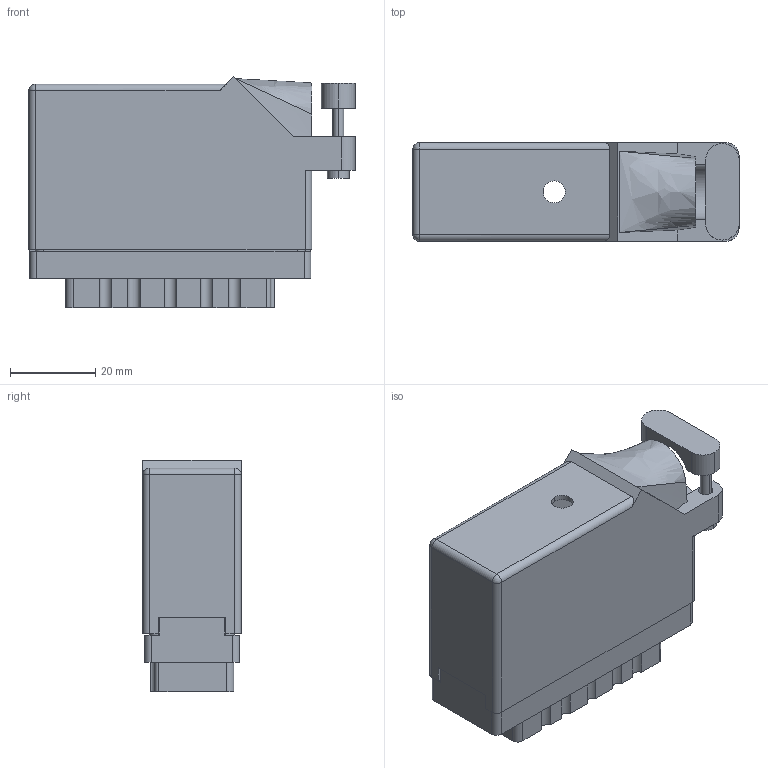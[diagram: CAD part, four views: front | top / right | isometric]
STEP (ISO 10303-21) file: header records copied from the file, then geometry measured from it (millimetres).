
FILE_DESCRIPTION (( 'STEP AP203' ), '1' );
FILE_NAME ('516-056-000-220.STEP', '2020-03-05T19:26:28', ( '' ), ( '' ), 'SwSTEP 2.0', 'SolidWorks 2016', '' );
FILE_SCHEMA (( 'CONFIG_CONTROL_DESIGN' ));
Length unit declared in the file: inch
Products named in the file (3): 516-056-000-220; 516-230-001_Plastic - 056 Side Entry; 516 Part Receptacle_056
Assembly tree (2 placements, depth 2):
  516-056-000-220
    516 Part Receptacle_056
    516-230-001_Plastic - 056 Side Entry
Bounding box: 76.5 x 23.11 x 54.15 mm (x, y, z)
Volume: 26495.7 mm3; surface area: 36846.7 mm2
Topology: 2 solids, 2 shells, 1337 faces, 3928 edges, 2614 vertices
Faces by surface type: plane 930, cylinder 400, bspline 3, cone 2, sphere 2
Entity records: 45130 total; most frequent: CARTESIAN_POINT 7975, ORIENTED_EDGE 7852, DIRECTION 7623, EDGE_CURVE 3926, LINE 2899, VECTOR 2899, VERTEX_POINT 2614, AXIS2_PLACEMENT_3D 2362
